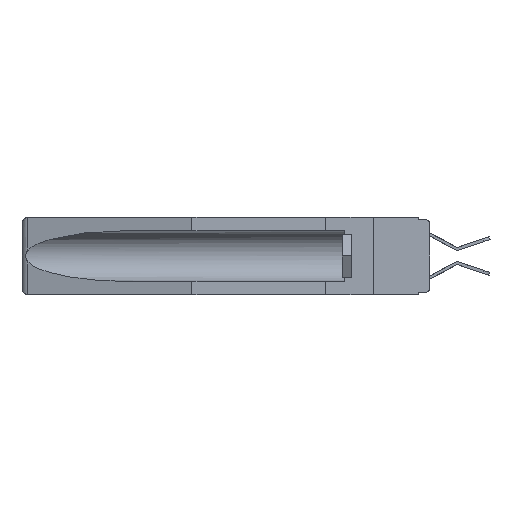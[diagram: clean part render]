
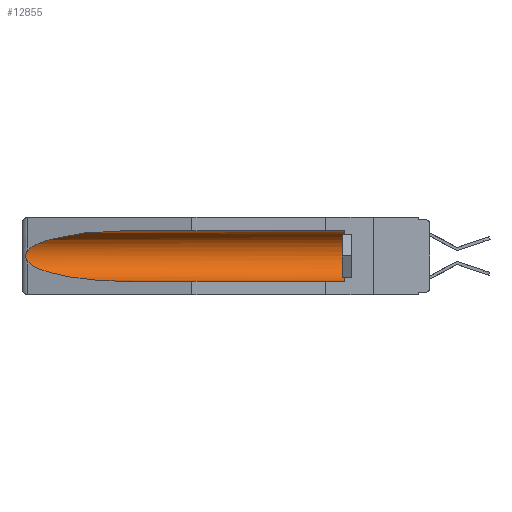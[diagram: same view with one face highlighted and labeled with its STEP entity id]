
A CAD part, left-side view. The second image highlights one B-rep face of the part: STEP entity #12855.
In plain terms, the highlighted cylindrical face has radius 2.857 mm (diameter 5.715 mm), a partial arc.
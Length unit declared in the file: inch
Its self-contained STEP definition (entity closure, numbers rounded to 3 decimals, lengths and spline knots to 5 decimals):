
#485 = CARTESIAN_POINT ( 'NONE',  ( 0.21114, 1.30732, -0.284 ) ) ;
#628 = LINE ( 'NONE', #11193, #10252 ) ;
#928 = CARTESIAN_POINT ( 'NONE',  ( 0.25451, 1.48313, -0.09465 ) ) ;
#1144 = CARTESIAN_POINT ( 'NONE',  ( 0.26537, 1.52718, -0.14972 ) ) ;
#1169 = AXIS2_PLACEMENT_3D ( 'NONE', #16138, #3586, #8149 ) ;
#1238 = ORIENTED_EDGE ( 'NONE', *, *, #9490, .T. ) ;
#1337 = CARTESIAN_POINT ( 'NONE',  ( 0.155, 0.126, -0.1715 ) ) ;
#1747 = DIRECTION ( 'NONE',  ( 0., 1., 0. ) ) ;
#1836 = VERTEX_POINT ( 'NONE', #2191 ) ;
#1892 = CARTESIAN_POINT ( 'NONE',  ( 0.26537, 1.52718, -0.19328 ) ) ;
#2011 = B_SPLINE_CURVE_WITH_KNOTS ( 'NONE', 3,
 ( #1144, #3085, #14135, #15769, #9522, #3211, #4305, #12098, #7355, #16927 ),
 .UNSPECIFIED., .F., .F.,
 ( 4, 2, 2, 2, 4 ),
 ( 0., 0.00029, 0.00058, 0.00087, 0.00117 ),
 .UNSPECIFIED. ) ;
#2066 = CARTESIAN_POINT ( 'NONE',  ( 0.155, 1.07973, -0.284 ) ) ;
#2191 = CARTESIAN_POINT ( 'NONE',  ( 0.155, 0.126, -0.059 ) ) ;
#2569 = EDGE_CURVE ( 'NONE', #12547, #6417, #18465, .T. ) ;
#2629 =( BOUNDED_CURVE ( )  B_SPLINE_CURVE ( 3, ( #1892, #11394, #485, #17742 ),
 .UNSPECIFIED., .F., .F. ) 
 B_SPLINE_CURVE_WITH_KNOTS ( ( 4, 4 ),
 ( 0.1948, 1.5708 ),
 .UNSPECIFIED. ) 
 CURVE ( )  GEOMETRIC_REPRESENTATION_ITEM ( )  RATIONAL_B_SPLINE_CURVE ( ( 1., 0.848, 0.848, 1. ) ) 
 REPRESENTATION_ITEM ( '' )  );
#2906 = FACE_OUTER_BOUND ( 'NONE', #12306, .T. ) ;
#3085 = CARTESIAN_POINT ( 'NONE',  ( 0.26597, 1.52961, -0.15275 ) ) ;
#3201 = CARTESIAN_POINT ( 'NONE',  ( 0.155, 1.07973, -0.059 ) ) ;
#3211 = CARTESIAN_POINT ( 'NONE',  ( 0.2675, 1.53308, -0.17534 ) ) ;
#3586 = DIRECTION ( 'NONE',  ( 0., 1., 0. ) ) ;
#4305 = CARTESIAN_POINT ( 'NONE',  ( 0.2673, 1.53269, -0.17917 ) ) ;
#5115 = ORIENTED_EDGE ( 'NONE', *, *, #2569, .F. ) ;
#5175 = CARTESIAN_POINT ( 'NONE',  ( 0.155, 1.07973, -0.059 ) ) ;
#5259 = EDGE_CURVE ( 'NONE', #14163, #8864, #13237, .T. ) ;
#5309 = AXIS2_PLACEMENT_3D ( 'NONE', #1337, #15330, #13662 ) ;
#6417 = VERTEX_POINT ( 'NONE', #2066 ) ;
#7031 = CARTESIAN_POINT ( 'NONE',  ( 0.155, -0.30754, -0.284 ) ) ;
#7260 = EDGE_CURVE ( 'NONE', #12547, #1836, #13292, .T. ) ;
#7281 = CARTESIAN_POINT ( 'NONE',  ( 0.26537, 1.52718, -0.14972 ) ) ;
#7355 = CARTESIAN_POINT ( 'NONE',  ( 0.26597, 1.5296, -0.19026 ) ) ;
#8149 = DIRECTION ( 'NONE',  ( 0., 0., 1. ) ) ;
#8176 = EDGE_CURVE ( 'NONE', #8864, #9904, #2011, .T. ) ;
#8694 = DIRECTION ( 'NONE',  ( 0., 1., 0. ) ) ;
#8864 = VERTEX_POINT ( 'NONE', #17467 ) ;
#9330 = CARTESIAN_POINT ( 'NONE',  ( 0.26537, 1.52718, -0.19328 ) ) ;
#9413 = EDGE_CURVE ( 'NONE', #1836, #14163, #628, .T. ) ;
#9490 = EDGE_CURVE ( 'NONE', #9904, #6417, #2629, .T. ) ;
#9522 = CARTESIAN_POINT ( 'NONE',  ( 0.2675, 1.53308, -0.16763 ) ) ;
#9844 = VECTOR ( 'NONE', #8694, 39.37008 ) ;
#9904 = VERTEX_POINT ( 'NONE', #9330 ) ;
#9918 = ORIENTED_EDGE ( 'NONE', *, *, #5259, .T. ) ;
#10038 = CARTESIAN_POINT ( 'NONE',  ( 0.21114, 1.30732, -0.059 ) ) ;
#10252 = VECTOR ( 'NONE', #1747, 39.37008 ) ;
#10805 = CYLINDRICAL_SURFACE ( 'NONE', #1169, 0.1125 ) ;
#11193 = CARTESIAN_POINT ( 'NONE',  ( 0.155, -0.30754, -0.059 ) ) ;
#11394 = CARTESIAN_POINT ( 'NONE',  ( 0.25451, 1.48313, -0.24835 ) ) ;
#11453 = CARTESIAN_POINT ( 'NONE',  ( 0.155, 0.126, -0.284 ) ) ;
#12098 = CARTESIAN_POINT ( 'NONE',  ( 0.26655, 1.53094, -0.18657 ) ) ;
#12203 = ORIENTED_EDGE ( 'NONE', *, *, #9413, .T. ) ;
#12306 = EDGE_LOOP ( 'NONE', ( #9918, #14841, #1238, #5115, #17817, #12203 ) ) ;
#12547 = VERTEX_POINT ( 'NONE', #11453 ) ;
#12855 = ADVANCED_FACE ( 'NONE', ( #2906 ), #10805, .F. ) ;
#13237 =( BOUNDED_CURVE ( )  B_SPLINE_CURVE ( 3, ( #5175, #10038, #928, #7281 ),
 .UNSPECIFIED., .F., .F. ) 
 B_SPLINE_CURVE_WITH_KNOTS ( ( 4, 4 ),
 ( 4.71239, 6.08839 ),
 .UNSPECIFIED. ) 
 CURVE ( )  GEOMETRIC_REPRESENTATION_ITEM ( )  RATIONAL_B_SPLINE_CURVE ( ( 1., 0.848, 0.848, 1. ) ) 
 REPRESENTATION_ITEM ( '' )  );
#13292 = CIRCLE ( 'NONE', #5309, 0.1125 ) ;
#13662 = DIRECTION ( 'NONE',  ( 0., 0., 1. ) ) ;
#14135 = CARTESIAN_POINT ( 'NONE',  ( 0.26654, 1.53092, -0.15636 ) ) ;
#14163 = VERTEX_POINT ( 'NONE', #3201 ) ;
#14841 = ORIENTED_EDGE ( 'NONE', *, *, #8176, .T. ) ;
#15330 = DIRECTION ( 'NONE',  ( 0., -1., 0. ) ) ;
#15769 = CARTESIAN_POINT ( 'NONE',  ( 0.2673, 1.5327, -0.16383 ) ) ;
#16138 = CARTESIAN_POINT ( 'NONE',  ( 0.155, -0.30754, -0.1715 ) ) ;
#16927 = CARTESIAN_POINT ( 'NONE',  ( 0.26537, 1.52718, -0.19328 ) ) ;
#17467 = CARTESIAN_POINT ( 'NONE',  ( 0.26537, 1.52718, -0.14972 ) ) ;
#17742 = CARTESIAN_POINT ( 'NONE',  ( 0.155, 1.07973, -0.284 ) ) ;
#17817 = ORIENTED_EDGE ( 'NONE', *, *, #7260, .T. ) ;
#18465 = LINE ( 'NONE', #7031, #9844 ) ;
